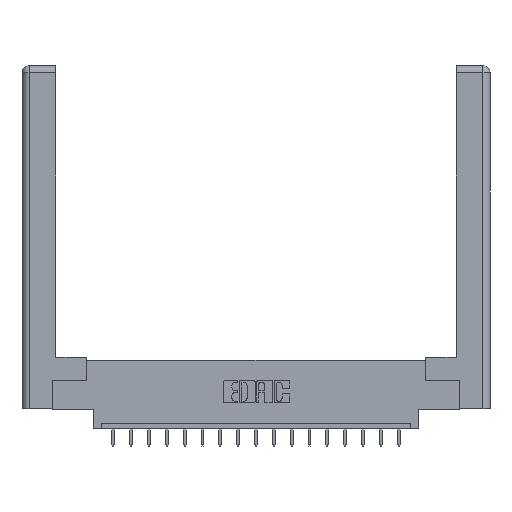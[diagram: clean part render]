
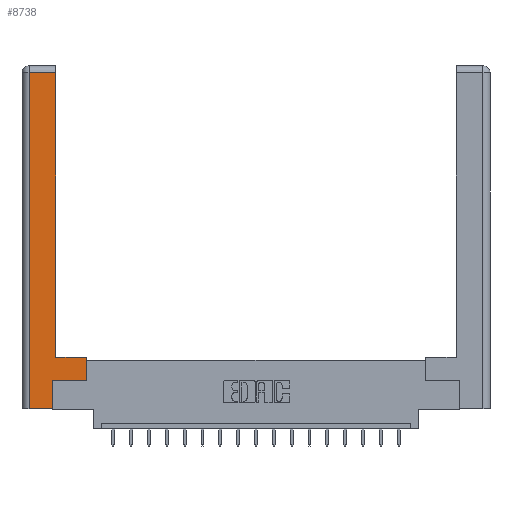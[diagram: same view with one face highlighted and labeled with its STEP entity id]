
A CAD part, top view. The second image highlights one B-rep face of the part: STEP entity #8738.
In plain terms, the highlighted planar face has unit normal (0, 0, 1).
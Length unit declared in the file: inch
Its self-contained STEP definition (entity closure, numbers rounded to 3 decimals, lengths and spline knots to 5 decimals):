
#121 = DIRECTION ( 'NONE',  ( 0., 1., 0. ) ) ;
#153 = CARTESIAN_POINT ( 'NONE',  ( 0.295, 0.45, 0. ) ) ;
#382 = VERTEX_POINT ( 'NONE', #1753 ) ;
#768 = EDGE_CURVE ( 'NONE', #382, #16235, #12371, .T. ) ;
#940 = VECTOR ( 'NONE', #6555, 39.37008 ) ;
#949 = LINE ( 'NONE', #153, #16953 ) ;
#1466 = DIRECTION ( 'NONE',  ( 1., 0., 0. ) ) ;
#1539 = DIRECTION ( 'NONE',  ( 1., 0., 0. ) ) ;
#1686 = ORIENTED_EDGE ( 'NONE', *, *, #3447, .T. ) ;
#1753 = CARTESIAN_POINT ( 'NONE',  ( 0.295, 2.94, 0. ) ) ;
#1780 = DIRECTION ( 'NONE',  ( -1., 0., 0. ) ) ;
#1793 = LINE ( 'NONE', #4619, #5214 ) ;
#1807 = CARTESIAN_POINT ( 'NONE',  ( 0.565, 0.45, 0. ) ) ;
#2155 = CARTESIAN_POINT ( 'NONE',  ( 0.0615, 0., 0. ) ) ;
#2792 = VERTEX_POINT ( 'NONE', #2155 ) ;
#3248 = EDGE_CURVE ( 'NONE', #16235, #2792, #4303, .T. ) ;
#3409 = FACE_OUTER_BOUND ( 'NONE', #16552, .T. ) ;
#3447 = EDGE_CURVE ( 'NONE', #12978, #12185, #1793, .T. ) ;
#3854 = CARTESIAN_POINT ( 'NONE',  ( 0.265, 0., 0. ) ) ;
#4303 = LINE ( 'NONE', #14164, #9674 ) ;
#4619 = CARTESIAN_POINT ( 'NONE',  ( 0.565, 0.245, 0. ) ) ;
#5214 = VECTOR ( 'NONE', #1539, 39.37008 ) ;
#5610 = VECTOR ( 'NONE', #11335, 39.37008 ) ;
#5910 = EDGE_CURVE ( 'NONE', #2792, #7872, #11831, .T. ) ;
#6555 = DIRECTION ( 'NONE',  ( 0., 1., 0. ) ) ;
#6934 = EDGE_CURVE ( 'NONE', #18405, #10292, #949, .T. ) ;
#7482 = CARTESIAN_POINT ( 'NONE',  ( 0.265, 0., 0. ) ) ;
#7539 = DIRECTION ( 'NONE',  ( 0., 0., -1. ) ) ;
#7872 = VERTEX_POINT ( 'NONE', #3854 ) ;
#8738 = ADVANCED_FACE ( 'NONE', ( #3409 ), #17682, .F. ) ;
#9674 = VECTOR ( 'NONE', #10106, 39.37008 ) ;
#10106 = DIRECTION ( 'NONE',  ( 0., -1., 0. ) ) ;
#10226 = CARTESIAN_POINT ( 'NONE',  ( 0.295, 0.45, 0. ) ) ;
#10292 = VERTEX_POINT ( 'NONE', #10226 ) ;
#10741 = CARTESIAN_POINT ( 'NONE',  ( 0.265, 0.245, 0. ) ) ;
#11335 = DIRECTION ( 'NONE',  ( 0., 1., 0. ) ) ;
#11337 = ORIENTED_EDGE ( 'NONE', *, *, #17040, .T. ) ;
#11831 = LINE ( 'NONE', #7482, #13613 ) ;
#11941 = ORIENTED_EDGE ( 'NONE', *, *, #15782, .T. ) ;
#12068 = CARTESIAN_POINT ( 'NONE',  ( 0.565, 0.245, 0. ) ) ;
#12185 = VERTEX_POINT ( 'NONE', #12068 ) ;
#12223 = CARTESIAN_POINT ( 'NONE',  ( 0.295, 3., 0. ) ) ;
#12371 = LINE ( 'NONE', #12546, #15955 ) ;
#12546 = CARTESIAN_POINT ( 'NONE',  ( 0.0615, 2.94, 0. ) ) ;
#12628 = CARTESIAN_POINT ( 'NONE',  ( 0.565, 0.45, 0. ) ) ;
#12978 = VERTEX_POINT ( 'NONE', #13776 ) ;
#13425 = EDGE_CURVE ( 'NONE', #10292, #382, #17956, .T. ) ;
#13558 = AXIS2_PLACEMENT_3D ( 'NONE', #16106, #7539, #1780 ) ;
#13613 = VECTOR ( 'NONE', #1466, 39.37008 ) ;
#13776 = CARTESIAN_POINT ( 'NONE',  ( 0.265, 0.245, 0. ) ) ;
#14164 = CARTESIAN_POINT ( 'NONE',  ( 0.0615, 0., 0. ) ) ;
#15381 = VECTOR ( 'NONE', #121, 39.37008 ) ;
#15782 = EDGE_CURVE ( 'NONE', #12185, #18405, #17870, .T. ) ;
#15902 = ORIENTED_EDGE ( 'NONE', *, *, #3248, .T. ) ;
#15955 = VECTOR ( 'NONE', #18396, 39.37008 ) ;
#16106 = CARTESIAN_POINT ( 'NONE',  ( 0., 0., 0. ) ) ;
#16235 = VERTEX_POINT ( 'NONE', #18590 ) ;
#16269 = LINE ( 'NONE', #10741, #940 ) ;
#16456 = ORIENTED_EDGE ( 'NONE', *, *, #6934, .T. ) ;
#16552 = EDGE_LOOP ( 'NONE', ( #18484, #17338, #15902, #17724, #11337, #1686, #11941, #16456 ) ) ;
#16953 = VECTOR ( 'NONE', #17554, 39.37008 ) ;
#17040 = EDGE_CURVE ( 'NONE', #7872, #12978, #16269, .T. ) ;
#17338 = ORIENTED_EDGE ( 'NONE', *, *, #768, .T. ) ;
#17554 = DIRECTION ( 'NONE',  ( -1., 0., 0. ) ) ;
#17682 = PLANE ( 'NONE',  #13558 ) ;
#17724 = ORIENTED_EDGE ( 'NONE', *, *, #5910, .T. ) ;
#17870 = LINE ( 'NONE', #1807, #15381 ) ;
#17956 = LINE ( 'NONE', #12223, #5610 ) ;
#18396 = DIRECTION ( 'NONE',  ( -1., 0., 0. ) ) ;
#18405 = VERTEX_POINT ( 'NONE', #12628 ) ;
#18484 = ORIENTED_EDGE ( 'NONE', *, *, #13425, .T. ) ;
#18590 = CARTESIAN_POINT ( 'NONE',  ( 0.0615, 2.94, 0. ) ) ;
